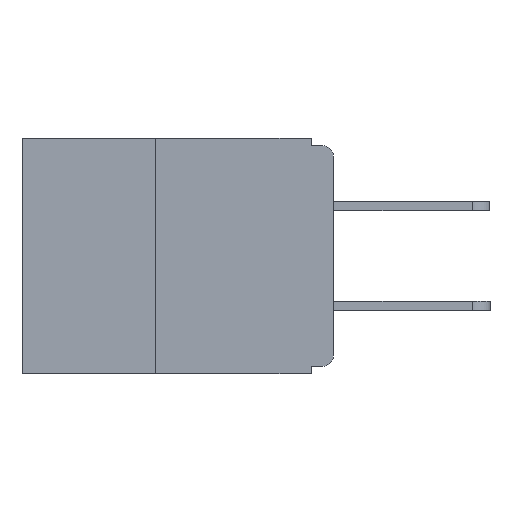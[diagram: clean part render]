
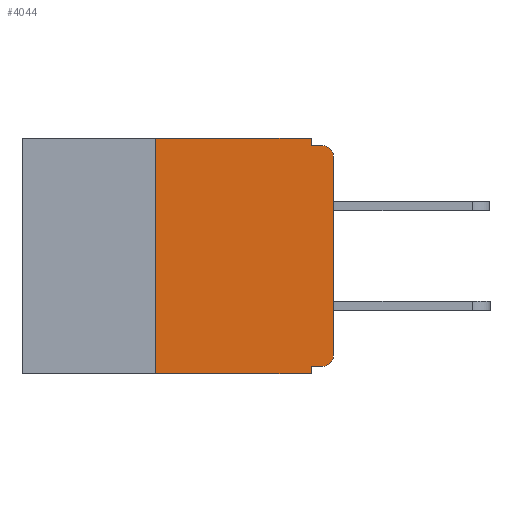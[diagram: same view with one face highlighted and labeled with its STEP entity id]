
A CAD part, left-side view. The second image highlights one B-rep face of the part: STEP entity #4044.
In plain terms, the highlighted planar face has unit normal (-1, 0, 0).
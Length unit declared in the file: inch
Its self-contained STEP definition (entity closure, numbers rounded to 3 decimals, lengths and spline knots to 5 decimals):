
#16 = VECTOR ( 'NONE', #7388, 39.37008 ) ;
#26 = EDGE_CURVE ( 'NONE', #8327, #5118, #9345, .T. ) ;
#40 = CARTESIAN_POINT ( 'NONE',  ( 0., 0.015, -0.32 ) ) ;
#123 = CARTESIAN_POINT ( 'NONE',  ( 0., 0.437, -0.33 ) ) ;
#174 = VECTOR ( 'NONE', #4731, 39.37008 ) ;
#692 = ORIENTED_EDGE ( 'NONE', *, *, #26, .F. ) ;
#796 = EDGE_CURVE ( 'NONE', #5118, #14116, #4791, .T. ) ;
#1144 = CARTESIAN_POINT ( 'NONE',  ( 0., 0.015, -0.305 ) ) ;
#1196 = EDGE_CURVE ( 'NONE', #13698, #5785, #5202, .T. ) ;
#1713 = CARTESIAN_POINT ( 'NONE',  ( 0., 0.25, -0.33 ) ) ;
#1748 = VECTOR ( 'NONE', #12906, 39.37008 ) ;
#2000 = VECTOR ( 'NONE', #14428, 39.37008 ) ;
#2007 = CARTESIAN_POINT ( 'NONE',  ( 0., 0.031, -0.33 ) ) ;
#2042 = FACE_OUTER_BOUND ( 'NONE', #2112, .T. ) ;
#2112 = EDGE_LOOP ( 'NONE', ( #4613, #7385, #7795, #11152, #2377, #12783, #11187, #5526, #692, #4484 ) ) ;
#2329 = VECTOR ( 'NONE', #15330, 39.37008 ) ;
#2353 = DIRECTION ( 'NONE',  ( 0., 0., -1. ) ) ;
#2377 = ORIENTED_EDGE ( 'NONE', *, *, #13150, .F. ) ;
#3390 = CARTESIAN_POINT ( 'NONE',  ( 0., 0.031, 0. ) ) ;
#4044 = ADVANCED_FACE ( 'NONE', ( #2042 ), #7296, .F. ) ;
#4484 = ORIENTED_EDGE ( 'NONE', *, *, #12646, .T. ) ;
#4613 = ORIENTED_EDGE ( 'NONE', *, *, #1196, .T. ) ;
#4731 = DIRECTION ( 'NONE',  ( 0., 0., -1. ) ) ;
#4791 = LINE ( 'NONE', #13811, #14652 ) ;
#5043 = CARTESIAN_POINT ( 'NONE',  ( 0., 0.015, -0.025 ) ) ;
#5118 = VERTEX_POINT ( 'NONE', #9943 ) ;
#5202 = LINE ( 'NONE', #16056, #1748 ) ;
#5208 = CARTESIAN_POINT ( 'NONE',  ( 0., 0.015, -0.01 ) ) ;
#5428 = CARTESIAN_POINT ( 'NONE',  ( 0., 0.437, 0. ) ) ;
#5526 = ORIENTED_EDGE ( 'NONE', *, *, #796, .F. ) ;
#5677 = VERTEX_POINT ( 'NONE', #13608 ) ;
#5785 = VERTEX_POINT ( 'NONE', #6140 ) ;
#6099 = CARTESIAN_POINT ( 'NONE',  ( 0., 0.031, -0.01 ) ) ;
#6140 = CARTESIAN_POINT ( 'NONE',  ( 0., 0., -0.025 ) ) ;
#6427 = DIRECTION ( 'NONE',  ( 0., 0., -1. ) ) ;
#6728 = DIRECTION ( 'NONE',  ( 0., 0., -1. ) ) ;
#6733 = DIRECTION ( 'NONE',  ( 1., 0., 0. ) ) ;
#7243 = CARTESIAN_POINT ( 'NONE',  ( 0., 0.437, 0. ) ) ;
#7296 = PLANE ( 'NONE',  #12627 ) ;
#7385 = ORIENTED_EDGE ( 'NONE', *, *, #7634, .T. ) ;
#7388 = DIRECTION ( 'NONE',  ( 0., 0., 1. ) ) ;
#7634 = EDGE_CURVE ( 'NONE', #5785, #16141, #14131, .T. ) ;
#7795 = ORIENTED_EDGE ( 'NONE', *, *, #11661, .F. ) ;
#8078 = EDGE_CURVE ( 'NONE', #11769, #11861, #13722, .T. ) ;
#8327 = VERTEX_POINT ( 'NONE', #40 ) ;
#9194 = DIRECTION ( 'NONE',  ( 0., -1., 0. ) ) ;
#9345 = LINE ( 'NONE', #11758, #2329 ) ;
#9871 = EDGE_CURVE ( 'NONE', #5677, #12514, #10463, .T. ) ;
#9897 = AXIS2_PLACEMENT_3D ( 'NONE', #1144, #10192, #2353 ) ;
#9943 = CARTESIAN_POINT ( 'NONE',  ( 0., 0.031, -0.32 ) ) ;
#10192 = DIRECTION ( 'NONE',  ( -1., 0., 0. ) ) ;
#10463 = LINE ( 'NONE', #3390, #174 ) ;
#11152 = ORIENTED_EDGE ( 'NONE', *, *, #9871, .F. ) ;
#11187 = ORIENTED_EDGE ( 'NONE', *, *, #11587, .T. ) ;
#11587 = EDGE_CURVE ( 'NONE', #11769, #14116, #12013, .T. ) ;
#11661 = EDGE_CURVE ( 'NONE', #12514, #16141, #14584, .T. ) ;
#11758 = CARTESIAN_POINT ( 'NONE',  ( 0., 0., -0.32 ) ) ;
#11769 = VERTEX_POINT ( 'NONE', #1713 ) ;
#11861 = VERTEX_POINT ( 'NONE', #14752 ) ;
#12013 = LINE ( 'NONE', #123, #15705 ) ;
#12514 = VERTEX_POINT ( 'NONE', #6099 ) ;
#12627 = AXIS2_PLACEMENT_3D ( 'NONE', #7243, #6733, #6728 ) ;
#12646 = EDGE_CURVE ( 'NONE', #8327, #13698, #13593, .T. ) ;
#12783 = ORIENTED_EDGE ( 'NONE', *, *, #8078, .F. ) ;
#12906 = DIRECTION ( 'NONE',  ( 0., 0., 1. ) ) ;
#13150 = EDGE_CURVE ( 'NONE', #11861, #5677, #15258, .T. ) ;
#13593 = CIRCLE ( 'NONE', #9897, 0.015 ) ;
#13608 = CARTESIAN_POINT ( 'NONE',  ( 0., 0.031, 0. ) ) ;
#13676 = AXIS2_PLACEMENT_3D ( 'NONE', #5043, #14070, #6427 ) ;
#13698 = VERTEX_POINT ( 'NONE', #15323 ) ;
#13722 = LINE ( 'NONE', #13733, #16 ) ;
#13733 = CARTESIAN_POINT ( 'NONE',  ( 0., 0.25, -0.33 ) ) ;
#13811 = CARTESIAN_POINT ( 'NONE',  ( 0., 0.031, -0.33 ) ) ;
#13816 = VECTOR ( 'NONE', #14402, 39.37008 ) ;
#14070 = DIRECTION ( 'NONE',  ( -1., 0., 0. ) ) ;
#14116 = VERTEX_POINT ( 'NONE', #2007 ) ;
#14131 = CIRCLE ( 'NONE', #13676, 0.015 ) ;
#14402 = DIRECTION ( 'NONE',  ( 0., -1., 0. ) ) ;
#14428 = DIRECTION ( 'NONE',  ( 0., -1., 0. ) ) ;
#14584 = LINE ( 'NONE', #15589, #13816 ) ;
#14652 = VECTOR ( 'NONE', #14725, 39.37008 ) ;
#14725 = DIRECTION ( 'NONE',  ( 0., 0., -1. ) ) ;
#14752 = CARTESIAN_POINT ( 'NONE',  ( 0., 0.25, 0. ) ) ;
#15258 = LINE ( 'NONE', #5428, #2000 ) ;
#15323 = CARTESIAN_POINT ( 'NONE',  ( 0., 0., -0.305 ) ) ;
#15330 = DIRECTION ( 'NONE',  ( 0., 1., 0. ) ) ;
#15589 = CARTESIAN_POINT ( 'NONE',  ( 0., 0., -0.01 ) ) ;
#15705 = VECTOR ( 'NONE', #9194, 39.37008 ) ;
#16056 = CARTESIAN_POINT ( 'NONE',  ( 0., 0., 0. ) ) ;
#16141 = VERTEX_POINT ( 'NONE', #5208 ) ;
